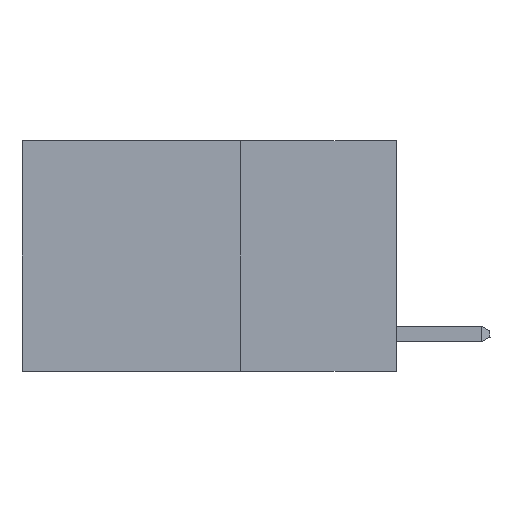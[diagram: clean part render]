
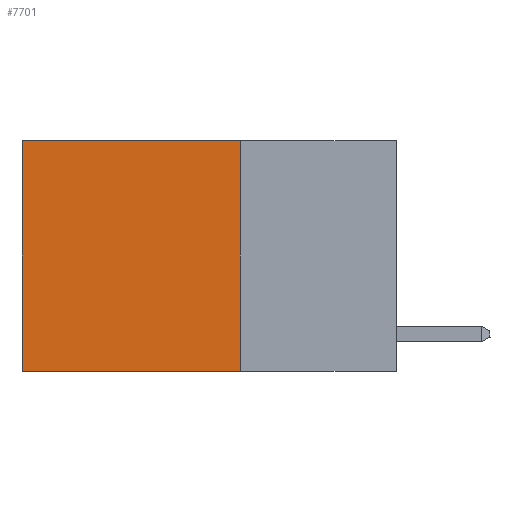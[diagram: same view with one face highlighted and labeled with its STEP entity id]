
A CAD part, left-side view. The second image highlights one B-rep face of the part: STEP entity #7701.
In plain terms, the highlighted planar face has unit normal (-1, 0, 0).
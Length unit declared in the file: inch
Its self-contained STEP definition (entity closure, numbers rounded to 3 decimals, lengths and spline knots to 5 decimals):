
#344 = ORIENTED_EDGE ( 'NONE', *, *, #7351, .F. ) ;
#352 = PLANE ( 'NONE',  #11975 ) ;
#810 = VERTEX_POINT ( 'NONE', #14180 ) ;
#1440 = ORIENTED_EDGE ( 'NONE', *, *, #10532, .T. ) ;
#1481 = CARTESIAN_POINT ( 'NONE',  ( 0.2625, 0.6, -0.37 ) ) ;
#2135 = ORIENTED_EDGE ( 'NONE', *, *, #8707, .T. ) ;
#2600 = DIRECTION ( 'NONE',  ( 1., 0., 0. ) ) ;
#3115 = CARTESIAN_POINT ( 'NONE',  ( 0.2625, 0.6, 0. ) ) ;
#3609 = CARTESIAN_POINT ( 'NONE',  ( 0.2625, 0.25, 0. ) ) ;
#4070 = LINE ( 'NONE', #3115, #14313 ) ;
#4227 = LINE ( 'NONE', #13247, #6622 ) ;
#4240 = ORIENTED_EDGE ( 'NONE', *, *, #8164, .F. ) ;
#4694 = LINE ( 'NONE', #3609, #12468 ) ;
#6012 = VERTEX_POINT ( 'NONE', #8611 ) ;
#6484 = DIRECTION ( 'NONE',  ( 0., 0., -1. ) ) ;
#6585 = DIRECTION ( 'NONE',  ( 0., 1., 0. ) ) ;
#6622 = VECTOR ( 'NONE', #6484, 39.37008 ) ;
#6695 = VERTEX_POINT ( 'NONE', #13671 ) ;
#7061 = VECTOR ( 'NONE', #13153, 39.37008 ) ;
#7097 = DIRECTION ( 'NONE',  ( 0., 0., -1. ) ) ;
#7351 = EDGE_CURVE ( 'NONE', #810, #11042, #9574, .T. ) ;
#7558 = EDGE_LOOP ( 'NONE', ( #2135, #344, #4240, #1440 ) ) ;
#7701 = ADVANCED_FACE ( 'NONE', ( #11548 ), #352, .F. ) ;
#8164 = EDGE_CURVE ( 'NONE', #6012, #810, #4227, .T. ) ;
#8611 = CARTESIAN_POINT ( 'NONE',  ( 0.2625, 0.25, 0. ) ) ;
#8707 = EDGE_CURVE ( 'NONE', #6695, #11042, #4070, .T. ) ;
#9574 = LINE ( 'NONE', #13013, #7061 ) ;
#10532 = EDGE_CURVE ( 'NONE', #6012, #6695, #4694, .T. ) ;
#11042 = VERTEX_POINT ( 'NONE', #1481 ) ;
#11548 = FACE_OUTER_BOUND ( 'NONE', #7558, .T. ) ;
#11975 = AXIS2_PLACEMENT_3D ( 'NONE', #12570, #2600, #7097 ) ;
#12468 = VECTOR ( 'NONE', #6585, 39.37008 ) ;
#12570 = CARTESIAN_POINT ( 'NONE',  ( 0.2625, 0.25, 0. ) ) ;
#13013 = CARTESIAN_POINT ( 'NONE',  ( 0.2625, 0.25, -0.37 ) ) ;
#13080 = DIRECTION ( 'NONE',  ( 0., 0., -1. ) ) ;
#13153 = DIRECTION ( 'NONE',  ( 0., 1., 0. ) ) ;
#13247 = CARTESIAN_POINT ( 'NONE',  ( 0.2625, 0.25, 0. ) ) ;
#13671 = CARTESIAN_POINT ( 'NONE',  ( 0.2625, 0.6, 0. ) ) ;
#14180 = CARTESIAN_POINT ( 'NONE',  ( 0.2625, 0.25, -0.37 ) ) ;
#14313 = VECTOR ( 'NONE', #13080, 39.37008 ) ;
